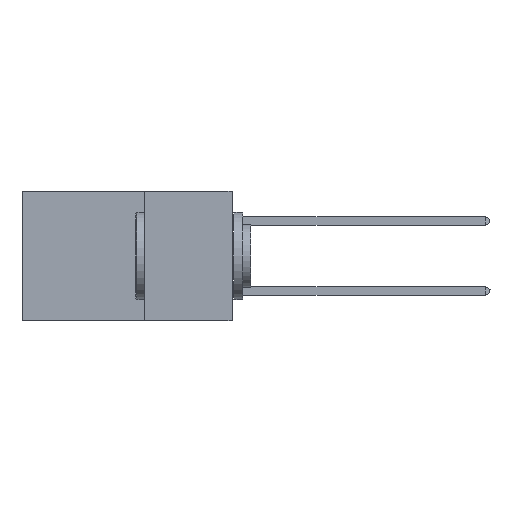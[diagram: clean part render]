
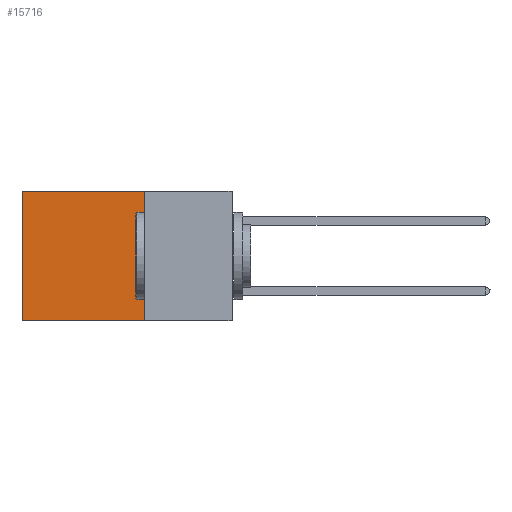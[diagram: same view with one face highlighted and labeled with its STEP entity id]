
A CAD part, left-side view. The second image highlights one B-rep face of the part: STEP entity #15716.
In plain terms, the highlighted planar face has unit normal (-1, 0, 0).
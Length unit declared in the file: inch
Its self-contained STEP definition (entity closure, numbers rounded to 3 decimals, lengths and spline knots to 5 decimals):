
#804 = EDGE_CURVE ( 'NONE', #17665, #12124, #5481, .T. ) ;
#835 = CARTESIAN_POINT ( 'NONE',  ( 0.2875, 0.25, -0.37 ) ) ;
#932 = PLANE ( 'NONE',  #15065 ) ;
#1905 = FACE_OUTER_BOUND ( 'NONE', #12062, .T. ) ;
#2649 = LINE ( 'NONE', #7357, #3322 ) ;
#3047 = CARTESIAN_POINT ( 'NONE',  ( 0.2875, 0.25, 0. ) ) ;
#3322 = VECTOR ( 'NONE', #9447, 39.37008 ) ;
#3643 = DIRECTION ( 'NONE',  ( 0., 1., 0. ) ) ;
#4191 = VECTOR ( 'NONE', #6222, 39.37008 ) ;
#5481 = LINE ( 'NONE', #24622, #4191 ) ;
#6222 = DIRECTION ( 'NONE',  ( 0., 0., -1. ) ) ;
#6365 = CARTESIAN_POINT ( 'NONE',  ( 0.2875, 0.6, 0. ) ) ;
#7357 = CARTESIAN_POINT ( 'NONE',  ( 0.2875, 0.25, 0. ) ) ;
#7724 = CARTESIAN_POINT ( 'NONE',  ( 0.2875, 0.25, -0.37 ) ) ;
#8765 = EDGE_CURVE ( 'NONE', #11208, #12124, #24209, .T. ) ;
#9447 = DIRECTION ( 'NONE',  ( 0., 1., 0. ) ) ;
#10960 = ORIENTED_EDGE ( 'NONE', *, *, #11871, .T. ) ;
#11208 = VERTEX_POINT ( 'NONE', #835 ) ;
#11413 = DIRECTION ( 'NONE',  ( 0., 0., -1. ) ) ;
#11871 = EDGE_CURVE ( 'NONE', #16361, #17665, #2649, .T. ) ;
#12062 = EDGE_LOOP ( 'NONE', ( #19805, #22309, #17942, #10960 ) ) ;
#12124 = VERTEX_POINT ( 'NONE', #26413 ) ;
#13513 = VECTOR ( 'NONE', #3643, 39.37008 ) ;
#15065 = AXIS2_PLACEMENT_3D ( 'NONE', #3047, #23562, #11413 ) ;
#15394 = CARTESIAN_POINT ( 'NONE',  ( 0.2875, 0.25, 0. ) ) ;
#15716 = ADVANCED_FACE ( 'NONE', ( #1905 ), #932, .F. ) ;
#16361 = VERTEX_POINT ( 'NONE', #17605 ) ;
#17458 = DIRECTION ( 'NONE',  ( 0., 0., -1. ) ) ;
#17605 = CARTESIAN_POINT ( 'NONE',  ( 0.2875, 0.25, 0. ) ) ;
#17665 = VERTEX_POINT ( 'NONE', #6365 ) ;
#17942 = ORIENTED_EDGE ( 'NONE', *, *, #20483, .F. ) ;
#19796 = VECTOR ( 'NONE', #17458, 39.37008 ) ;
#19805 = ORIENTED_EDGE ( 'NONE', *, *, #804, .T. ) ;
#20483 = EDGE_CURVE ( 'NONE', #16361, #11208, #25050, .T. ) ;
#22309 = ORIENTED_EDGE ( 'NONE', *, *, #8765, .F. ) ;
#23562 = DIRECTION ( 'NONE',  ( 1., 0., 0. ) ) ;
#24209 = LINE ( 'NONE', #7724, #13513 ) ;
#24622 = CARTESIAN_POINT ( 'NONE',  ( 0.2875, 0.6, 0. ) ) ;
#25050 = LINE ( 'NONE', #15394, #19796 ) ;
#26413 = CARTESIAN_POINT ( 'NONE',  ( 0.2875, 0.6, -0.37 ) ) ;
